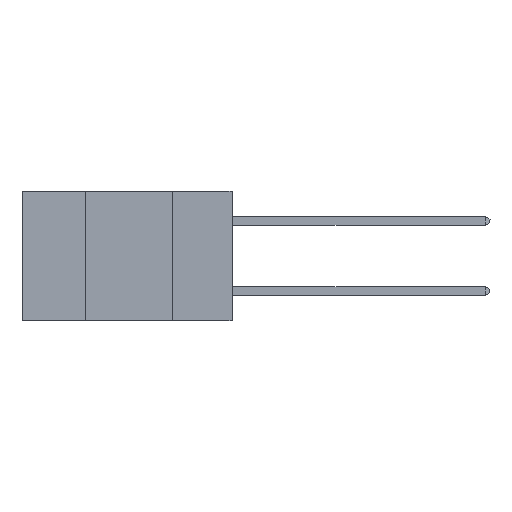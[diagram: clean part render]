
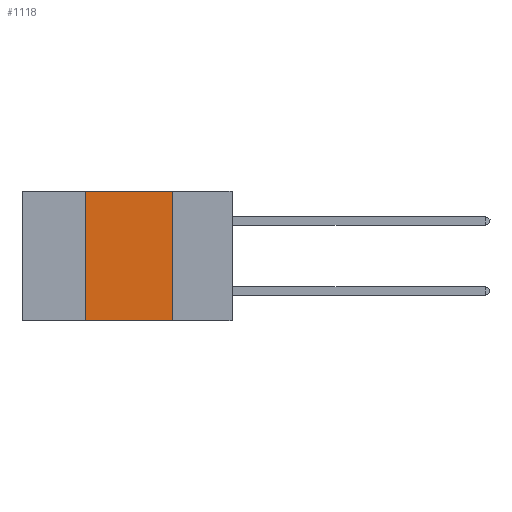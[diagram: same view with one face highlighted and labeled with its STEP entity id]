
A CAD part, left-side view. The second image highlights one B-rep face of the part: STEP entity #1118.
In plain terms, the highlighted planar face has unit normal (-1, 0, 0).
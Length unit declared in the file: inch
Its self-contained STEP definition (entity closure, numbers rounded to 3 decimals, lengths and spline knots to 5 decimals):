
#130 = EDGE_CURVE ( 'NONE', #11259, #5943, #11325, .T. ) ;
#659 = PLANE ( 'NONE',  #2084 ) ;
#1118 = ADVANCED_FACE ( 'NONE', ( #10234 ), #659, .F. ) ;
#1135 = CARTESIAN_POINT ( 'NONE',  ( 0., 0.6, 0. ) ) ;
#1707 = CARTESIAN_POINT ( 'NONE',  ( 0., 0.17, 0. ) ) ;
#1876 = VECTOR ( 'NONE', #10239, 39.37008 ) ;
#2084 = AXIS2_PLACEMENT_3D ( 'NONE', #13475, #8130, #9592 ) ;
#2225 = CARTESIAN_POINT ( 'NONE',  ( 0., 0.17, -0.37 ) ) ;
#2269 = VERTEX_POINT ( 'NONE', #2225 ) ;
#2279 = EDGE_CURVE ( 'NONE', #11259, #2269, #8447, .T. ) ;
#2763 = LINE ( 'NONE', #1707, #1876 ) ;
#3050 = DIRECTION ( 'NONE',  ( 0., -1., 0. ) ) ;
#3108 = EDGE_CURVE ( 'NONE', #9995, #2269, #2763, .T. ) ;
#3472 = CARTESIAN_POINT ( 'NONE',  ( 0., 0.42, 0. ) ) ;
#3850 = EDGE_LOOP ( 'NONE', ( #8735, #10595, #9309, #7258 ) ) ;
#5024 = VECTOR ( 'NONE', #8251, 39.37008 ) ;
#5943 = VERTEX_POINT ( 'NONE', #3472 ) ;
#6265 = EDGE_CURVE ( 'NONE', #5943, #9995, #8281, .T. ) ;
#6478 = CARTESIAN_POINT ( 'NONE',  ( 0., 0.17, 0. ) ) ;
#7258 = ORIENTED_EDGE ( 'NONE', *, *, #2279, .T. ) ;
#8130 = DIRECTION ( 'NONE',  ( 1., 0., 0. ) ) ;
#8251 = DIRECTION ( 'NONE',  ( 0., 0., 1. ) ) ;
#8281 = LINE ( 'NONE', #1135, #13342 ) ;
#8447 = LINE ( 'NONE', #10689, #13490 ) ;
#8735 = ORIENTED_EDGE ( 'NONE', *, *, #3108, .F. ) ;
#9309 = ORIENTED_EDGE ( 'NONE', *, *, #130, .F. ) ;
#9592 = DIRECTION ( 'NONE',  ( 0., 0., -1. ) ) ;
#9995 = VERTEX_POINT ( 'NONE', #6478 ) ;
#10213 = CARTESIAN_POINT ( 'NONE',  ( 0., 0.42, -0.37 ) ) ;
#10234 = FACE_OUTER_BOUND ( 'NONE', #3850, .T. ) ;
#10239 = DIRECTION ( 'NONE',  ( 0., 0., -1. ) ) ;
#10424 = CARTESIAN_POINT ( 'NONE',  ( 0., 0.42, 0. ) ) ;
#10595 = ORIENTED_EDGE ( 'NONE', *, *, #6265, .F. ) ;
#10623 = DIRECTION ( 'NONE',  ( 0., -1., 0. ) ) ;
#10689 = CARTESIAN_POINT ( 'NONE',  ( 0., 0.6, -0.37 ) ) ;
#11259 = VERTEX_POINT ( 'NONE', #10213 ) ;
#11325 = LINE ( 'NONE', #10424, #5024 ) ;
#13342 = VECTOR ( 'NONE', #3050, 39.37008 ) ;
#13475 = CARTESIAN_POINT ( 'NONE',  ( 0., 0.6, 0. ) ) ;
#13490 = VECTOR ( 'NONE', #10623, 39.37008 ) ;
